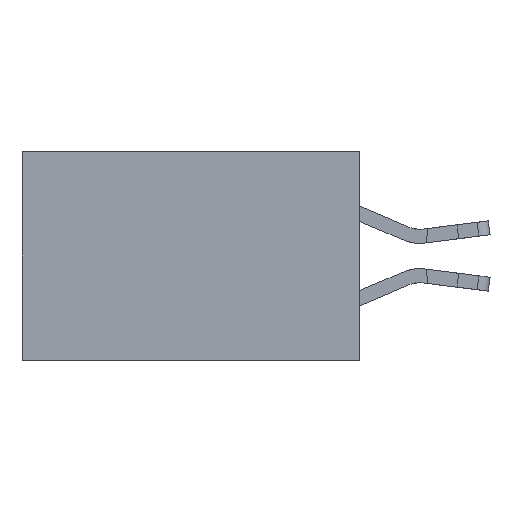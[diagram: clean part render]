
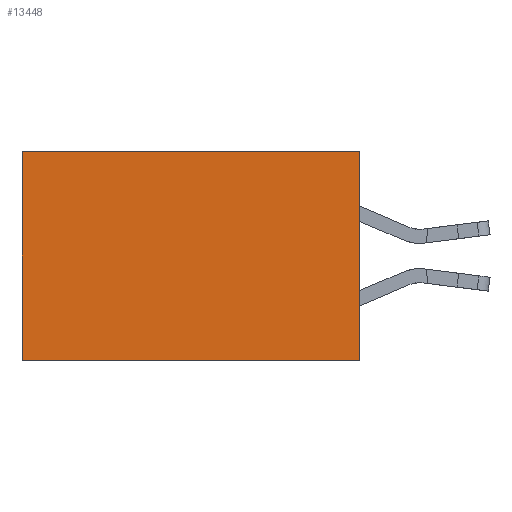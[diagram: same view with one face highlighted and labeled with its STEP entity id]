
A CAD part, left-side view. The second image highlights one B-rep face of the part: STEP entity #13448.
In plain terms, the highlighted planar face has unit normal (-1, 0, 0).
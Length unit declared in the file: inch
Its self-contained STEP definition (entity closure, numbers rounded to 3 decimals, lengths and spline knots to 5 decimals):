
#438 = CARTESIAN_POINT ( 'NONE',  ( 0.2875, 0., 0. ) ) ;
#1081 = EDGE_CURVE ( 'NONE', #10511, #2474, #8951, .T. ) ;
#1441 = DIRECTION ( 'NONE',  ( 0., 0., -1. ) ) ;
#1961 = ORIENTED_EDGE ( 'NONE', *, *, #3023, .F. ) ;
#2033 = EDGE_CURVE ( 'NONE', #12030, #10511, #6433, .T. ) ;
#2166 = DIRECTION ( 'NONE',  ( 0., 0., -1. ) ) ;
#2474 = VERTEX_POINT ( 'NONE', #13268 ) ;
#3023 = EDGE_CURVE ( 'NONE', #21605, #2474, #7736, .T. ) ;
#3204 = DIRECTION ( 'NONE',  ( 1., 0., 0. ) ) ;
#3210 = CARTESIAN_POINT ( 'NONE',  ( 0.2875, 0., -0.37 ) ) ;
#4424 = AXIS2_PLACEMENT_3D ( 'NONE', #20538, #3204, #1441 ) ;
#6271 = DIRECTION ( 'NONE',  ( 0., 1., 0. ) ) ;
#6278 = DIRECTION ( 'NONE',  ( 0., 0., -1. ) ) ;
#6433 = LINE ( 'NONE', #21349, #10556 ) ;
#7011 = VECTOR ( 'NONE', #2166, 39.37008 ) ;
#7736 = LINE ( 'NONE', #3210, #14634 ) ;
#8001 = ORIENTED_EDGE ( 'NONE', *, *, #1081, .T. ) ;
#8951 = LINE ( 'NONE', #22022, #17757 ) ;
#10080 = EDGE_CURVE ( 'NONE', #12030, #21605, #16629, .T. ) ;
#10511 = VERTEX_POINT ( 'NONE', #20702 ) ;
#10556 = VECTOR ( 'NONE', #6271, 39.37008 ) ;
#10868 = ORIENTED_EDGE ( 'NONE', *, *, #10080, .F. ) ;
#11847 = PLANE ( 'NONE',  #4424 ) ;
#12030 = VERTEX_POINT ( 'NONE', #438 ) ;
#12423 = CARTESIAN_POINT ( 'NONE',  ( 0.2875, 0., 0. ) ) ;
#13268 = CARTESIAN_POINT ( 'NONE',  ( 0.2875, 0.6, -0.37 ) ) ;
#13448 = ADVANCED_FACE ( 'NONE', ( #16993 ), #11847, .F. ) ;
#14634 = VECTOR ( 'NONE', #18666, 39.37008 ) ;
#14959 = CARTESIAN_POINT ( 'NONE',  ( 0.2875, 0., -0.37 ) ) ;
#16629 = LINE ( 'NONE', #12423, #7011 ) ;
#16661 = EDGE_LOOP ( 'NONE', ( #8001, #1961, #10868, #20722 ) ) ;
#16993 = FACE_OUTER_BOUND ( 'NONE', #16661, .T. ) ;
#17757 = VECTOR ( 'NONE', #6278, 39.37008 ) ;
#18666 = DIRECTION ( 'NONE',  ( 0., 1., 0. ) ) ;
#20538 = CARTESIAN_POINT ( 'NONE',  ( 0.2875, 0., 0. ) ) ;
#20702 = CARTESIAN_POINT ( 'NONE',  ( 0.2875, 0.6, 0. ) ) ;
#20722 = ORIENTED_EDGE ( 'NONE', *, *, #2033, .T. ) ;
#21349 = CARTESIAN_POINT ( 'NONE',  ( 0.2875, 0., 0. ) ) ;
#21605 = VERTEX_POINT ( 'NONE', #14959 ) ;
#22022 = CARTESIAN_POINT ( 'NONE',  ( 0.2875, 0.6, 0. ) ) ;
